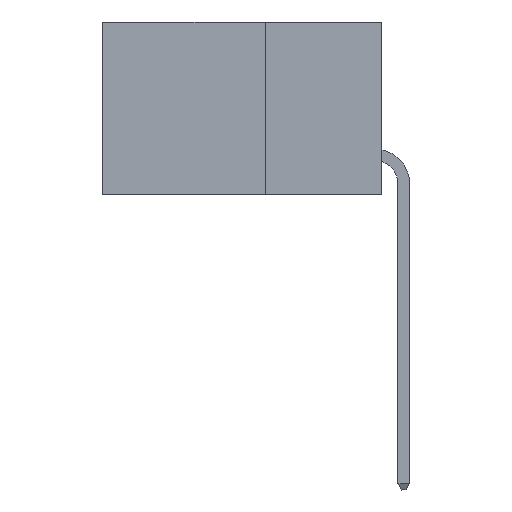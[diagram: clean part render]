
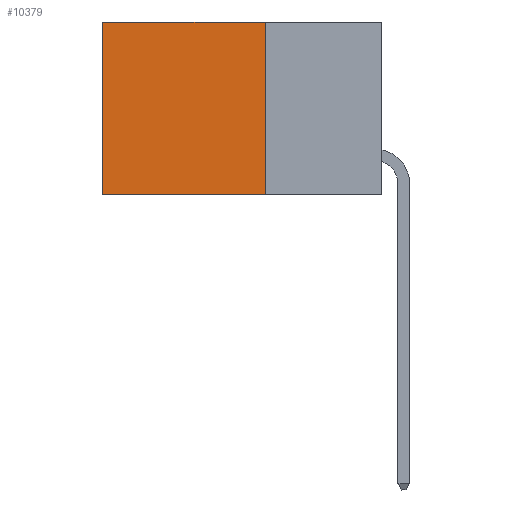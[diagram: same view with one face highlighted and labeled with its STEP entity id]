
A CAD part, left-side view. The second image highlights one B-rep face of the part: STEP entity #10379.
In plain terms, the highlighted planar face has unit normal (-1, 0, 0).
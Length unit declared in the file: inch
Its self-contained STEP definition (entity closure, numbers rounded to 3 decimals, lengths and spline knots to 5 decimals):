
#276 = LINE ( 'NONE', #14103, #3458 ) ;
#349 = AXIS2_PLACEMENT_3D ( 'NONE', #10205, #8905, #797 ) ;
#604 = DIRECTION ( 'NONE',  ( 0., 0., -1. ) ) ;
#681 = VECTOR ( 'NONE', #2838, 39.37008 ) ;
#797 = DIRECTION ( 'NONE',  ( 0., 0., -1. ) ) ;
#2107 = VERTEX_POINT ( 'NONE', #7739 ) ;
#2641 = VECTOR ( 'NONE', #2901, 39.37008 ) ;
#2838 = DIRECTION ( 'NONE',  ( 0., 1., 0. ) ) ;
#2901 = DIRECTION ( 'NONE',  ( 0., 0., -1. ) ) ;
#3458 = VECTOR ( 'NONE', #604, 39.37008 ) ;
#3486 = EDGE_CURVE ( 'NONE', #8895, #7084, #276, .T. ) ;
#4003 = VERTEX_POINT ( 'NONE', #11202 ) ;
#5432 = DIRECTION ( 'NONE',  ( 0., 1., 0. ) ) ;
#6611 = ORIENTED_EDGE ( 'NONE', *, *, #12589, .T. ) ;
#7084 = VERTEX_POINT ( 'NONE', #10445 ) ;
#7538 = PLANE ( 'NONE',  #349 ) ;
#7739 = CARTESIAN_POINT ( 'NONE',  ( 0.2875, 0.6, 0. ) ) ;
#7882 = EDGE_CURVE ( 'NONE', #2107, #4003, #16568, .T. ) ;
#7890 = LINE ( 'NONE', #16340, #681 ) ;
#8035 = ORIENTED_EDGE ( 'NONE', *, *, #7882, .T. ) ;
#8895 = VERTEX_POINT ( 'NONE', #13044 ) ;
#8905 = DIRECTION ( 'NONE',  ( 1., 0., 0. ) ) ;
#9088 = EDGE_CURVE ( 'NONE', #7084, #4003, #11713, .T. ) ;
#10205 = CARTESIAN_POINT ( 'NONE',  ( 0.2875, 0.25, 0. ) ) ;
#10309 = ORIENTED_EDGE ( 'NONE', *, *, #9088, .F. ) ;
#10379 = ADVANCED_FACE ( 'NONE', ( #11230 ), #7538, .F. ) ;
#10445 = CARTESIAN_POINT ( 'NONE',  ( 0.2875, 0.25, -0.37 ) ) ;
#11202 = CARTESIAN_POINT ( 'NONE',  ( 0.2875, 0.6, -0.37 ) ) ;
#11230 = FACE_OUTER_BOUND ( 'NONE', #11979, .T. ) ;
#11713 = LINE ( 'NONE', #13523, #15269 ) ;
#11979 = EDGE_LOOP ( 'NONE', ( #8035, #10309, #17315, #6611 ) ) ;
#12589 = EDGE_CURVE ( 'NONE', #8895, #2107, #7890, .T. ) ;
#13044 = CARTESIAN_POINT ( 'NONE',  ( 0.2875, 0.25, 0. ) ) ;
#13523 = CARTESIAN_POINT ( 'NONE',  ( 0.2875, 0.25, -0.37 ) ) ;
#13735 = CARTESIAN_POINT ( 'NONE',  ( 0.2875, 0.6, 0. ) ) ;
#14103 = CARTESIAN_POINT ( 'NONE',  ( 0.2875, 0.25, 0. ) ) ;
#15269 = VECTOR ( 'NONE', #5432, 39.37008 ) ;
#16340 = CARTESIAN_POINT ( 'NONE',  ( 0.2875, 0.25, 0. ) ) ;
#16568 = LINE ( 'NONE', #13735, #2641 ) ;
#17315 = ORIENTED_EDGE ( 'NONE', *, *, #3486, .F. ) ;
